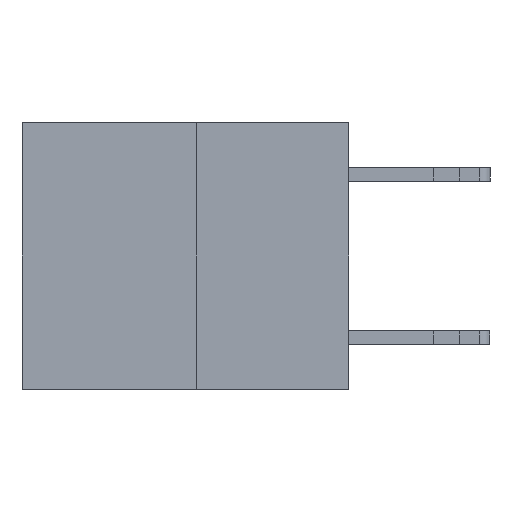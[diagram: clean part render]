
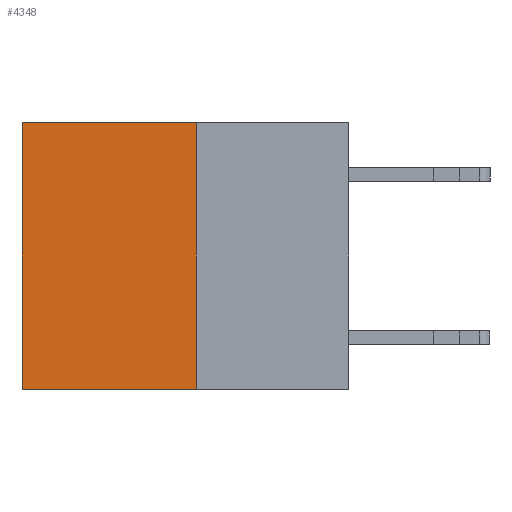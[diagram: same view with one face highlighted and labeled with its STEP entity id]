
A CAD part, left-side view. The second image highlights one B-rep face of the part: STEP entity #4348.
In plain terms, the highlighted planar face has unit normal (-1, 0, 0).
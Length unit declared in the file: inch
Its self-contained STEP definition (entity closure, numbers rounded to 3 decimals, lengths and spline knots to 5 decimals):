
#871 = DIRECTION ( 'NONE',  ( 0., 1., 0. ) ) ;
#918 = LINE ( 'NONE', #14951, #15757 ) ;
#1927 = EDGE_CURVE ( 'NONE', #18050, #13748, #16473, .T. ) ;
#3250 = CARTESIAN_POINT ( 'NONE',  ( 0.3165, 0.6, 0. ) ) ;
#3294 = CARTESIAN_POINT ( 'NONE',  ( 0.3165, 0.6, -0.49 ) ) ;
#3750 = CARTESIAN_POINT ( 'NONE',  ( 0.3165, 0.28, -0.49 ) ) ;
#4348 = ADVANCED_FACE ( 'NONE', ( #4648 ), #8647, .F. ) ;
#4648 = FACE_OUTER_BOUND ( 'NONE', #6539, .T. ) ;
#4869 = VERTEX_POINT ( 'NONE', #3250 ) ;
#5343 = DIRECTION ( 'NONE',  ( 0., 1., 0. ) ) ;
#6539 = EDGE_LOOP ( 'NONE', ( #18004, #15490, #13039, #12488 ) ) ;
#7628 = DIRECTION ( 'NONE',  ( 0., 0., -1. ) ) ;
#8224 = VERTEX_POINT ( 'NONE', #12222 ) ;
#8647 = PLANE ( 'NONE',  #13071 ) ;
#9695 = LINE ( 'NONE', #3294, #13060 ) ;
#10234 = DIRECTION ( 'NONE',  ( 0., 0., -1. ) ) ;
#10267 = EDGE_CURVE ( 'NONE', #8224, #18050, #918, .T. ) ;
#11063 = VECTOR ( 'NONE', #871, 39.37008 ) ;
#12222 = CARTESIAN_POINT ( 'NONE',  ( 0.3165, 0.28, 0. ) ) ;
#12488 = ORIENTED_EDGE ( 'NONE', *, *, #16476, .T. ) ;
#13039 = ORIENTED_EDGE ( 'NONE', *, *, #10267, .F. ) ;
#13060 = VECTOR ( 'NONE', #14621, 39.37008 ) ;
#13071 = AXIS2_PLACEMENT_3D ( 'NONE', #16811, #19331, #7628 ) ;
#13748 = VERTEX_POINT ( 'NONE', #14491 ) ;
#14491 = CARTESIAN_POINT ( 'NONE',  ( 0.3165, 0.6, -0.49 ) ) ;
#14621 = DIRECTION ( 'NONE',  ( 0., 0., -1. ) ) ;
#14794 = EDGE_CURVE ( 'NONE', #4869, #13748, #9695, .T. ) ;
#14951 = CARTESIAN_POINT ( 'NONE',  ( 0.3165, 0.28, -0.49 ) ) ;
#15490 = ORIENTED_EDGE ( 'NONE', *, *, #1927, .F. ) ;
#15757 = VECTOR ( 'NONE', #10234, 39.37008 ) ;
#15769 = VECTOR ( 'NONE', #5343, 39.37008 ) ;
#16473 = LINE ( 'NONE', #3750, #15769 ) ;
#16476 = EDGE_CURVE ( 'NONE', #8224, #4869, #19208, .T. ) ;
#16811 = CARTESIAN_POINT ( 'NONE',  ( 0.3165, 0.28, -0.49 ) ) ;
#17978 = CARTESIAN_POINT ( 'NONE',  ( 0.3165, 0.28, -0.49 ) ) ;
#18004 = ORIENTED_EDGE ( 'NONE', *, *, #14794, .T. ) ;
#18050 = VERTEX_POINT ( 'NONE', #17978 ) ;
#19208 = LINE ( 'NONE', #19356, #11063 ) ;
#19331 = DIRECTION ( 'NONE',  ( 1., 0., 0. ) ) ;
#19356 = CARTESIAN_POINT ( 'NONE',  ( 0.3165, 0.28, 0. ) ) ;
